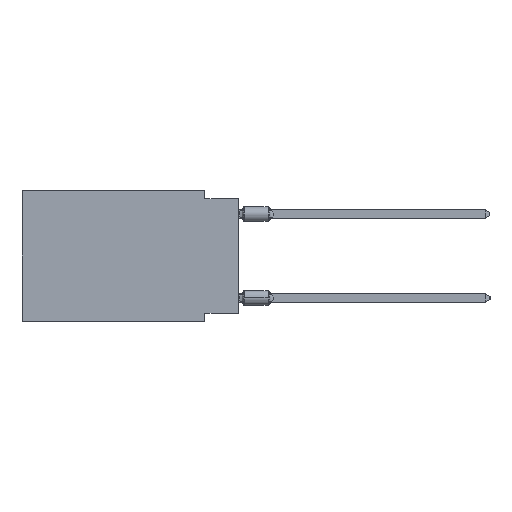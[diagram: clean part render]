
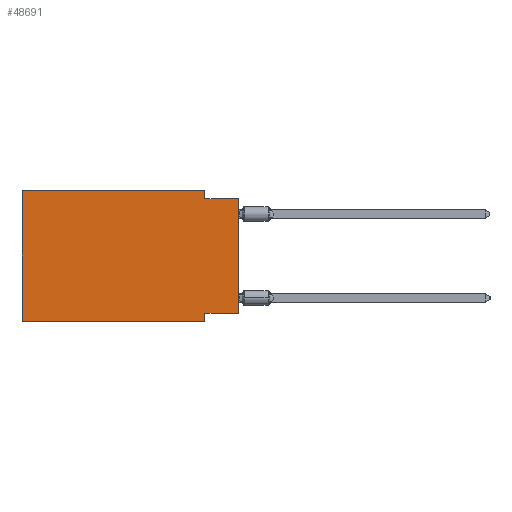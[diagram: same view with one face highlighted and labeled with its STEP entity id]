
A CAD part, left-side view. The second image highlights one B-rep face of the part: STEP entity #48691.
In plain terms, the highlighted planar face has unit normal (-1, 0, 0).
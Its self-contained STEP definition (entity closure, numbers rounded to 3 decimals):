
#496 = VERTEX_POINT ( 'NONE', #25496 ) ;
#712 = CARTESIAN_POINT ( 'NONE',  ( 0., 2.54, 0. ) ) ;
#4203 = LINE ( 'NONE', #52482, #30314 ) ;
#4280 = LINE ( 'NONE', #23414, #26452 ) ;
#5132 = DIRECTION ( 'NONE',  ( 0., -1., 0. ) ) ;
#5757 = ORIENTED_EDGE ( 'NONE', *, *, #24073, .F. ) ;
#6954 = FACE_OUTER_BOUND ( 'NONE', #17608, .T. ) ;
#8326 = LINE ( 'NONE', #31872, #45983 ) ;
#9420 = ORIENTED_EDGE ( 'NONE', *, *, #15269, .F. ) ;
#9457 = VERTEX_POINT ( 'NONE', #33261 ) ;
#9670 = LINE ( 'NONE', #33207, #62036 ) ;
#10374 = EDGE_CURVE ( 'NONE', #57223, #27339, #9670, .T. ) ;
#13327 = CARTESIAN_POINT ( 'NONE',  ( 0., 2.54, -9.906 ) ) ;
#14996 = VECTOR ( 'NONE', #48926, 1000. ) ;
#15050 = LINE ( 'NONE', #18903, #14996 ) ;
#15269 = EDGE_CURVE ( 'NONE', #27339, #9457, #4203, .T. ) ;
#15337 = EDGE_CURVE ( 'NONE', #17173, #496, #52800, .T. ) ;
#15712 = CARTESIAN_POINT ( 'NONE',  ( 0., 0., -9.271 ) ) ;
#17173 = VERTEX_POINT ( 'NONE', #15712 ) ;
#17608 = EDGE_LOOP ( 'NONE', ( #30837, #9420, #45812, #32950, #5757, #31935, #57901, #25941 ) ) ;
#17644 = VERTEX_POINT ( 'NONE', #13327 ) ;
#18625 = DIRECTION ( 'NONE',  ( 0., 1., 0. ) ) ;
#18903 = CARTESIAN_POINT ( 'NONE',  ( 0., 16.383, 0. ) ) ;
#21334 = VECTOR ( 'NONE', #18625, 1000. ) ;
#22028 = CARTESIAN_POINT ( 'NONE',  ( 0., 2.54, -0.635 ) ) ;
#23324 = DIRECTION ( 'NONE',  ( 0., 0., 1. ) ) ;
#23414 = CARTESIAN_POINT ( 'NONE',  ( 0., 16.383, 0. ) ) ;
#23447 = VERTEX_POINT ( 'NONE', #25315 ) ;
#23644 = EDGE_CURVE ( 'NONE', #25966, #17644, #8326, .T. ) ;
#24073 = EDGE_CURVE ( 'NONE', #25966, #23447, #15050, .T. ) ;
#24260 = VECTOR ( 'NONE', #23324, 1000. ) ;
#24652 = DIRECTION ( 'NONE',  ( 0., 0., -1. ) ) ;
#25315 = CARTESIAN_POINT ( 'NONE',  ( 0., 16.383, 0. ) ) ;
#25496 = CARTESIAN_POINT ( 'NONE',  ( 0., 2.54, -9.271 ) ) ;
#25790 = DIRECTION ( 'NONE',  ( 1., 0., 0. ) ) ;
#25941 = ORIENTED_EDGE ( 'NONE', *, *, #15337, .F. ) ;
#25966 = VERTEX_POINT ( 'NONE', #51563 ) ;
#26408 = PLANE ( 'NONE',  #38676 ) ;
#26452 = VECTOR ( 'NONE', #28123, 1000. ) ;
#27101 = EDGE_CURVE ( 'NONE', #17173, #9457, #61920, .T. ) ;
#27339 = VERTEX_POINT ( 'NONE', #22028 ) ;
#28123 = DIRECTION ( 'NONE',  ( 0., -1., 0. ) ) ;
#28817 = DIRECTION ( 'NONE',  ( 0., 0., -1. ) ) ;
#30314 = VECTOR ( 'NONE', #5132, 1000. ) ;
#30837 = ORIENTED_EDGE ( 'NONE', *, *, #27101, .T. ) ;
#31872 = CARTESIAN_POINT ( 'NONE',  ( 0., 16.383, -9.906 ) ) ;
#31935 = ORIENTED_EDGE ( 'NONE', *, *, #23644, .T. ) ;
#32950 = ORIENTED_EDGE ( 'NONE', *, *, #50689, .F. ) ;
#33207 = CARTESIAN_POINT ( 'NONE',  ( 0., 2.54, 0. ) ) ;
#33261 = CARTESIAN_POINT ( 'NONE',  ( 0., 0., -0.635 ) ) ;
#34888 = CARTESIAN_POINT ( 'NONE',  ( 0., 16.383, 0. ) ) ;
#37759 = CARTESIAN_POINT ( 'NONE',  ( 0., 0., -9.271 ) ) ;
#37834 = CARTESIAN_POINT ( 'NONE',  ( 0., 2.54, -9.906 ) ) ;
#38676 = AXIS2_PLACEMENT_3D ( 'NONE', #34888, #25790, #50248 ) ;
#38759 = LINE ( 'NONE', #37834, #44067 ) ;
#39569 = EDGE_CURVE ( 'NONE', #496, #17644, #38759, .T. ) ;
#44067 = VECTOR ( 'NONE', #24652, 1000. ) ;
#45812 = ORIENTED_EDGE ( 'NONE', *, *, #10374, .F. ) ;
#45983 = VECTOR ( 'NONE', #46602, 1000. ) ;
#46602 = DIRECTION ( 'NONE',  ( 0., -1., 0. ) ) ;
#48691 = ADVANCED_FACE ( 'NONE', ( #6954 ), #26408, .F. ) ;
#48926 = DIRECTION ( 'NONE',  ( 0., 0., 1. ) ) ;
#50248 = DIRECTION ( 'NONE',  ( 0., 0., -1. ) ) ;
#50689 = EDGE_CURVE ( 'NONE', #23447, #57223, #4280, .T. ) ;
#51563 = CARTESIAN_POINT ( 'NONE',  ( 0., 16.383, -9.906 ) ) ;
#52482 = CARTESIAN_POINT ( 'NONE',  ( 0., 0., -0.635 ) ) ;
#52800 = LINE ( 'NONE', #37759, #21334 ) ;
#57223 = VERTEX_POINT ( 'NONE', #712 ) ;
#57901 = ORIENTED_EDGE ( 'NONE', *, *, #39569, .F. ) ;
#61010 = CARTESIAN_POINT ( 'NONE',  ( 0., 0., 0. ) ) ;
#61920 = LINE ( 'NONE', #61010, #24260 ) ;
#62036 = VECTOR ( 'NONE', #28817, 1000. ) ;
